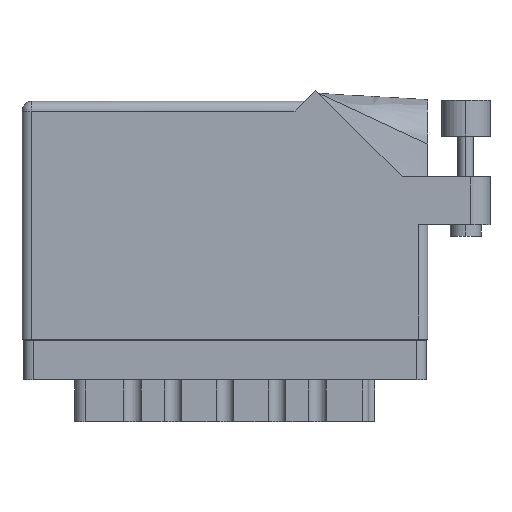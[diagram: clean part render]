
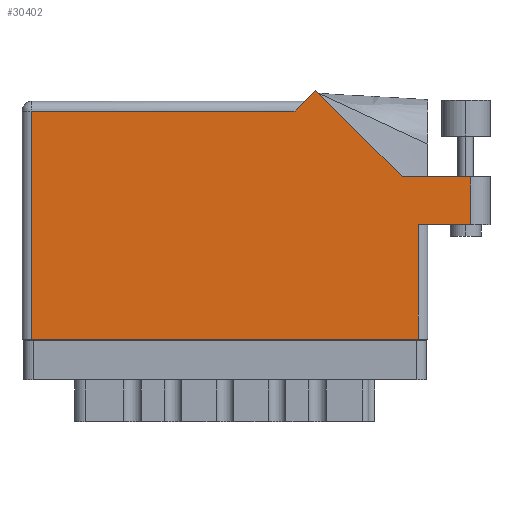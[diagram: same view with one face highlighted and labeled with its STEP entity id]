
A CAD part, front view. The second image highlights one B-rep face of the part: STEP entity #30402.
In plain terms, the highlighted face is planar.
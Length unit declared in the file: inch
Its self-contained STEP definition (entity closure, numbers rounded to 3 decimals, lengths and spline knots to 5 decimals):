
#509 = CARTESIAN_POINT ( 'NONE',  ( 2.887, 1.044, 0. ) ) ;
#1408 = CARTESIAN_POINT ( 'NONE',  ( 0., 0., 0. ) ) ;
#1639 = CARTESIAN_POINT ( 'NONE',  ( 1.757, 1.468, 0. ) ) ;
#1828 = ORIENTED_EDGE ( 'NONE', *, *, #9492, .T. ) ;
#2389 = VECTOR ( 'NONE', #40280, 39.37008 ) ;
#2921 = VECTOR ( 'NONE', #50240, 39.37008 ) ;
#2962 = EDGE_LOOP ( 'NONE', ( #11480, #28613, #49765, #33090, #1828, #28299, #28561, #9560, #15042 ) ) ;
#3554 = VECTOR ( 'NONE', #27246, 39.37008 ) ;
#4004 = CARTESIAN_POINT ( 'NONE',  ( 2.887, 1.044, 0. ) ) ;
#5257 = EDGE_CURVE ( 'NONE', #23469, #40761, #33667, .T. ) ;
#9492 = EDGE_CURVE ( 'NONE', #44003, #10830, #14713, .T. ) ;
#9560 = ORIENTED_EDGE ( 'NONE', *, *, #16176, .T. ) ;
#10054 = EDGE_CURVE ( 'NONE', #37956, #44003, #12689, .T. ) ;
#10597 = VECTOR ( 'NONE', #40794, 39.37008 ) ;
#10830 = VERTEX_POINT ( 'NONE', #1639 ) ;
#11184 = CARTESIAN_POINT ( 'NONE',  ( 0., 1.53, 0. ) ) ;
#11480 = ORIENTED_EDGE ( 'NONE', *, *, #5257, .T. ) ;
#11653 = EDGE_CURVE ( 'NONE', #47059, #37956, #25516, .T. ) ;
#12648 = CARTESIAN_POINT ( 'NONE',  ( 0., 1.468, 0. ) ) ;
#12689 = LINE ( 'NONE', #51779, #47023 ) ;
#14713 = LINE ( 'NONE', #52582, #2389 ) ;
#14911 = DIRECTION ( 'NONE',  ( -0.707, 0.707, 0. ) ) ;
#15042 = ORIENTED_EDGE ( 'NONE', *, *, #17714, .T. ) ;
#15430 = CARTESIAN_POINT ( 'NONE',  ( 0.062, 0., 0. ) ) ;
#16024 = CARTESIAN_POINT ( 'NONE',  ( 3.012, 1.044, 0. ) ) ;
#16176 = EDGE_CURVE ( 'NONE', #16968, #26819, #22528, .T. ) ;
#16968 = VERTEX_POINT ( 'NONE', #15430 ) ;
#17714 = EDGE_CURVE ( 'NONE', #26819, #23469, #33980, .T. ) ;
#18623 = CARTESIAN_POINT ( 'NONE',  ( 2.44642, 1.044, 0. ) ) ;
#20423 = CARTESIAN_POINT ( 'NONE',  ( 2.55, 0.737, 0. ) ) ;
#21140 = EDGE_CURVE ( 'NONE', #10830, #30957, #45335, .T. ) ;
#22242 = LINE ( 'NONE', #4004, #24844 ) ;
#22528 = LINE ( 'NONE', #1408, #31564 ) ;
#22629 = VECTOR ( 'NONE', #52081, 39.37008 ) ;
#23469 = VERTEX_POINT ( 'NONE', #36458 ) ;
#24844 = VECTOR ( 'NONE', #36547, 39.37008 ) ;
#25516 = LINE ( 'NONE', #16024, #10597 ) ;
#26819 = VERTEX_POINT ( 'NONE', #53395 ) ;
#26825 = FACE_OUTER_BOUND ( 'NONE', #2962, .T. ) ;
#27246 = DIRECTION ( 'NONE',  ( 0., -1., 0. ) ) ;
#28251 = EDGE_CURVE ( 'NONE', #30957, #16968, #41722, .T. ) ;
#28299 = ORIENTED_EDGE ( 'NONE', *, *, #21140, .T. ) ;
#28561 = ORIENTED_EDGE ( 'NONE', *, *, #28251, .T. ) ;
#28613 = ORIENTED_EDGE ( 'NONE', *, *, #42264, .T. ) ;
#30202 = DIRECTION ( 'NONE',  ( 1., 0., 0. ) ) ;
#30402 = ADVANCED_FACE ( 'NONE', ( #26825 ), #35802, .F. ) ;
#30957 = VERTEX_POINT ( 'NONE', #41299 ) ;
#31564 = VECTOR ( 'NONE', #30202, 39.37008 ) ;
#32394 = CARTESIAN_POINT ( 'NONE',  ( 1.88971, 1.60071, 0. ) ) ;
#32414 = VECTOR ( 'NONE', #41747, 39.37008 ) ;
#33090 = ORIENTED_EDGE ( 'NONE', *, *, #10054, .T. ) ;
#33667 = LINE ( 'NONE', #42301, #22629 ) ;
#33980 = LINE ( 'NONE', #20423, #2921 ) ;
#34889 = AXIS2_PLACEMENT_3D ( 'NONE', #11184, #44091, #48106 ) ;
#35802 = PLANE ( 'NONE',  #34889 ) ;
#36139 = CARTESIAN_POINT ( 'NONE',  ( 2.887, 0.737, 0. ) ) ;
#36458 = CARTESIAN_POINT ( 'NONE',  ( 2.55, 0.737, 0. ) ) ;
#36547 = DIRECTION ( 'NONE',  ( 0., 1., 0. ) ) ;
#37956 = VERTEX_POINT ( 'NONE', #18623 ) ;
#39333 = CARTESIAN_POINT ( 'NONE',  ( 0.062, 0., 0. ) ) ;
#40280 = DIRECTION ( 'NONE',  ( -0.707, -0.707, 0. ) ) ;
#40761 = VERTEX_POINT ( 'NONE', #36139 ) ;
#40794 = DIRECTION ( 'NONE',  ( -1., 0., 0. ) ) ;
#41299 = CARTESIAN_POINT ( 'NONE',  ( 0.062, 1.468, 0. ) ) ;
#41722 = LINE ( 'NONE', #39333, #3554 ) ;
#41747 = DIRECTION ( 'NONE',  ( -1., 0., 0. ) ) ;
#42264 = EDGE_CURVE ( 'NONE', #40761, #47059, #22242, .T. ) ;
#42301 = CARTESIAN_POINT ( 'NONE',  ( 2.612, 0.737, 0. ) ) ;
#44003 = VERTEX_POINT ( 'NONE', #32394 ) ;
#44091 = DIRECTION ( 'NONE',  ( 0., 0., -1. ) ) ;
#45335 = LINE ( 'NONE', #12648, #32414 ) ;
#47023 = VECTOR ( 'NONE', #14911, 39.37008 ) ;
#47059 = VERTEX_POINT ( 'NONE', #509 ) ;
#48106 = DIRECTION ( 'NONE',  ( -1., 0., 0. ) ) ;
#49765 = ORIENTED_EDGE ( 'NONE', *, *, #11653, .T. ) ;
#50240 = DIRECTION ( 'NONE',  ( 0., 1., 0. ) ) ;
#51779 = CARTESIAN_POINT ( 'NONE',  ( 2.44642, 1.044, 0. ) ) ;
#52081 = DIRECTION ( 'NONE',  ( 1., 0., 0. ) ) ;
#52582 = CARTESIAN_POINT ( 'NONE',  ( 1.819, 1.53, 0. ) ) ;
#53395 = CARTESIAN_POINT ( 'NONE',  ( 2.55, 0., 0. ) ) ;
